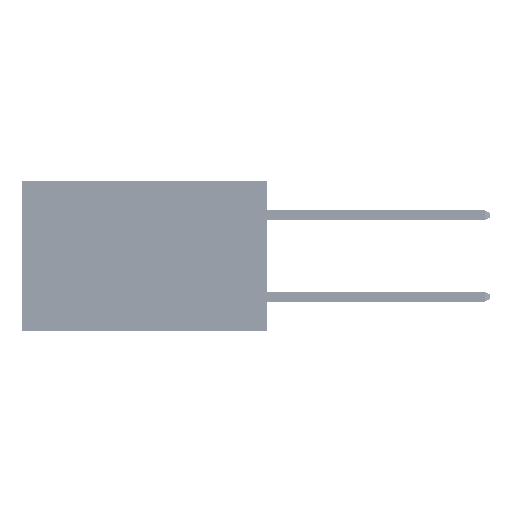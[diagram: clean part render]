
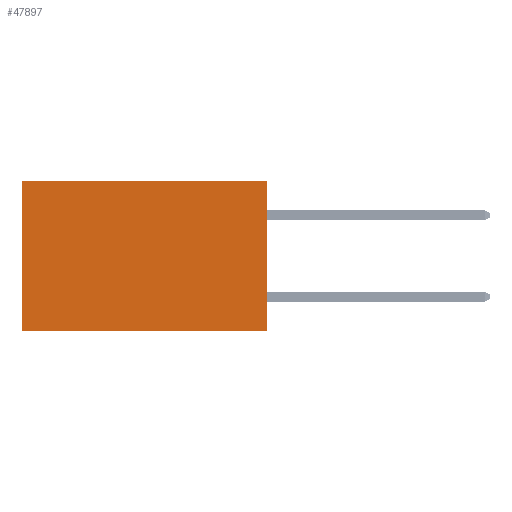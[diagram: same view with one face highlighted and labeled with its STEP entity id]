
A CAD part, left-side view. The second image highlights one B-rep face of the part: STEP entity #47897.
In plain terms, the highlighted planar face has unit normal (-1, 0, 0).
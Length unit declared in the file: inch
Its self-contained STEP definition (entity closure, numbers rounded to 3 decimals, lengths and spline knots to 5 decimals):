
#1976 = VECTOR ( 'NONE', #35541, 39.37008 ) ;
#2096 = CARTESIAN_POINT ( 'NONE',  ( 0.2875, 0., 0. ) ) ;
#4034 = ORIENTED_EDGE ( 'NONE', *, *, #40012, .F. ) ;
#4576 = VERTEX_POINT ( 'NONE', #29080 ) ;
#7080 = VERTEX_POINT ( 'NONE', #37992 ) ;
#9167 = AXIS2_PLACEMENT_3D ( 'NONE', #2096, #37677, #14007 ) ;
#11851 = CARTESIAN_POINT ( 'NONE',  ( 0.2875, 0., -0.37 ) ) ;
#12209 = DIRECTION ( 'NONE',  ( 0., 0., -1. ) ) ;
#12581 = ORIENTED_EDGE ( 'NONE', *, *, #30102, .T. ) ;
#14007 = DIRECTION ( 'NONE',  ( 0., 0., -1. ) ) ;
#16933 = CARTESIAN_POINT ( 'NONE',  ( 0.2875, 0.6, 0. ) ) ;
#18042 = FACE_OUTER_BOUND ( 'NONE', #27326, .T. ) ;
#18718 = CARTESIAN_POINT ( 'NONE',  ( 0.2875, 0., 0. ) ) ;
#18917 = LINE ( 'NONE', #16933, #38653 ) ;
#18929 = CARTESIAN_POINT ( 'NONE',  ( 0.2875, 0.6, -0.37 ) ) ;
#20012 = CARTESIAN_POINT ( 'NONE',  ( 0.2875, 0., 0. ) ) ;
#21778 = LINE ( 'NONE', #11851, #1976 ) ;
#24140 = LINE ( 'NONE', #20012, #33433 ) ;
#24887 = DIRECTION ( 'NONE',  ( 0., 0., -1. ) ) ;
#27326 = EDGE_LOOP ( 'NONE', ( #30898, #28625, #4034, #12581 ) ) ;
#28625 = ORIENTED_EDGE ( 'NONE', *, *, #34365, .F. ) ;
#28959 = LINE ( 'NONE', #18718, #48576 ) ;
#29080 = CARTESIAN_POINT ( 'NONE',  ( 0.2875, 0., 0. ) ) ;
#29735 = PLANE ( 'NONE',  #9167 ) ;
#30102 = EDGE_CURVE ( 'NONE', #4576, #7080, #28959, .T. ) ;
#30898 = ORIENTED_EDGE ( 'NONE', *, *, #45912, .T. ) ;
#33433 = VECTOR ( 'NONE', #12209, 39.37008 ) ;
#34365 = EDGE_CURVE ( 'NONE', #44888, #47437, #21778, .T. ) ;
#34438 = DIRECTION ( 'NONE',  ( 0., 1., 0. ) ) ;
#35541 = DIRECTION ( 'NONE',  ( 0., 1., 0. ) ) ;
#35988 = CARTESIAN_POINT ( 'NONE',  ( 0.2875, 0., -0.37 ) ) ;
#37677 = DIRECTION ( 'NONE',  ( 1., 0., 0. ) ) ;
#37992 = CARTESIAN_POINT ( 'NONE',  ( 0.2875, 0.6, 0. ) ) ;
#38653 = VECTOR ( 'NONE', #24887, 39.37008 ) ;
#40012 = EDGE_CURVE ( 'NONE', #4576, #44888, #24140, .T. ) ;
#44888 = VERTEX_POINT ( 'NONE', #35988 ) ;
#45912 = EDGE_CURVE ( 'NONE', #7080, #47437, #18917, .T. ) ;
#47437 = VERTEX_POINT ( 'NONE', #18929 ) ;
#47897 = ADVANCED_FACE ( 'NONE', ( #18042 ), #29735, .F. ) ;
#48576 = VECTOR ( 'NONE', #34438, 39.37008 ) ;
